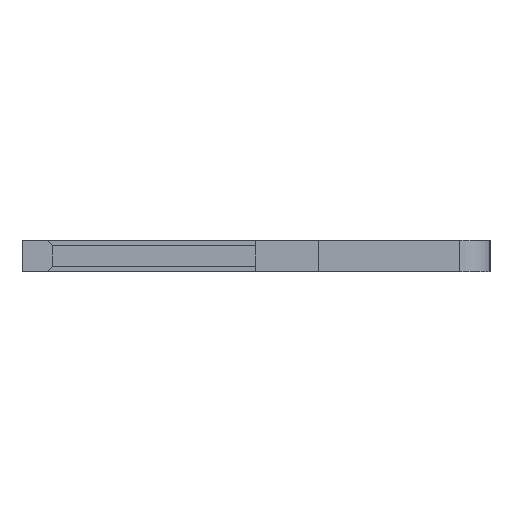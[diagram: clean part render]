
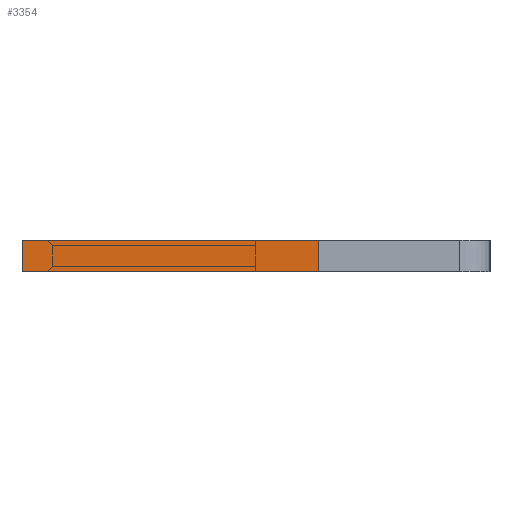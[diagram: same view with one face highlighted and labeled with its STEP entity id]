
A CAD part, left-side view. The second image highlights one B-rep face of the part: STEP entity #3354.
In plain terms, the highlighted face is planar.
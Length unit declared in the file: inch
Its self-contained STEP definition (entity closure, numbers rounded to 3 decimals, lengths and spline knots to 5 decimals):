
#50 = LINE ( 'NONE', #1362, #3309 ) ;
#260 = VERTEX_POINT ( 'NONE', #644 ) ;
#399 = FACE_OUTER_BOUND ( 'NONE', #3497, .T. ) ;
#439 = DIRECTION ( 'NONE',  ( 0., 1., 0. ) ) ;
#616 = EDGE_CURVE ( 'NONE', #736, #260, #3838, .T. ) ;
#644 = CARTESIAN_POINT ( 'NONE',  ( -0.01, 0.15, -0.04 ) ) ;
#736 = VERTEX_POINT ( 'NONE', #3122 ) ;
#791 = CARTESIAN_POINT ( 'NONE',  ( -0.01, -0.04, -0.04 ) ) ;
#819 = CARTESIAN_POINT ( 'NONE',  ( 0.01, -0.04, -0.04 ) ) ;
#826 = ORIENTED_EDGE ( 'NONE', *, *, #1850, .T. ) ;
#866 = VECTOR ( 'NONE', #2967, 39.37008 ) ;
#871 = PLANE ( 'NONE',  #3204 ) ;
#932 = DIRECTION ( 'NONE',  ( -1., 0., 0. ) ) ;
#1147 = LINE ( 'NONE', #1352, #866 ) ;
#1352 = CARTESIAN_POINT ( 'NONE',  ( 0.01, -0.04, -0.04 ) ) ;
#1362 = CARTESIAN_POINT ( 'NONE',  ( 0.01, 0.15, -0.04 ) ) ;
#1843 = VERTEX_POINT ( 'NONE', #791 ) ;
#1850 = EDGE_CURVE ( 'NONE', #3105, #1843, #1147, .T. ) ;
#1952 = LINE ( 'NONE', #3548, #2268 ) ;
#1975 = EDGE_CURVE ( 'NONE', #3105, #736, #50, .T. ) ;
#2219 = VECTOR ( 'NONE', #932, 39.37008 ) ;
#2246 = EDGE_CURVE ( 'NONE', #1843, #260, #1952, .T. ) ;
#2268 = VECTOR ( 'NONE', #2592, 39.37008 ) ;
#2514 = CARTESIAN_POINT ( 'NONE',  ( 0.01, 0.15, -0.04 ) ) ;
#2592 = DIRECTION ( 'NONE',  ( 0., 1., 0. ) ) ;
#2967 = DIRECTION ( 'NONE',  ( -1., 0., 0. ) ) ;
#3056 = CARTESIAN_POINT ( 'NONE',  ( 0.01, 0.15, -0.04 ) ) ;
#3082 = DIRECTION ( 'NONE',  ( 1., 0., 0. ) ) ;
#3105 = VERTEX_POINT ( 'NONE', #819 ) ;
#3122 = CARTESIAN_POINT ( 'NONE',  ( 0.01, 0.15, -0.04 ) ) ;
#3204 = AXIS2_PLACEMENT_3D ( 'NONE', #3056, #3405, #3082 ) ;
#3216 = ORIENTED_EDGE ( 'NONE', *, *, #1975, .F. ) ;
#3309 = VECTOR ( 'NONE', #439, 39.37008 ) ;
#3354 = ADVANCED_FACE ( 'NONE', ( #399 ), #871, .F. ) ;
#3405 = DIRECTION ( 'NONE',  ( 0., 0., 1. ) ) ;
#3497 = EDGE_LOOP ( 'NONE', ( #3550, #3796, #3216, #826 ) ) ;
#3548 = CARTESIAN_POINT ( 'NONE',  ( -0.01, 0.15, -0.04 ) ) ;
#3550 = ORIENTED_EDGE ( 'NONE', *, *, #2246, .T. ) ;
#3796 = ORIENTED_EDGE ( 'NONE', *, *, #616, .F. ) ;
#3838 = LINE ( 'NONE', #2514, #2219 ) ;
